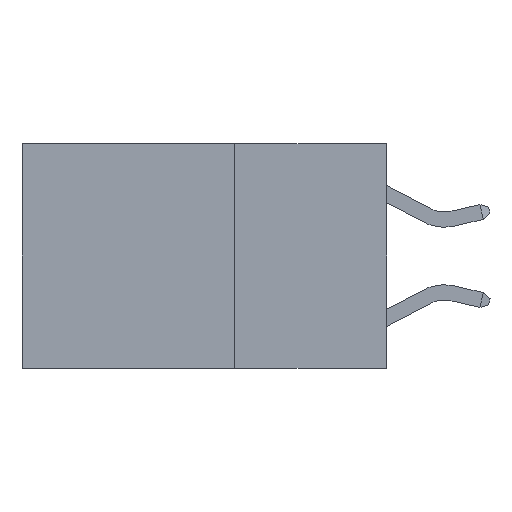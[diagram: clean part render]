
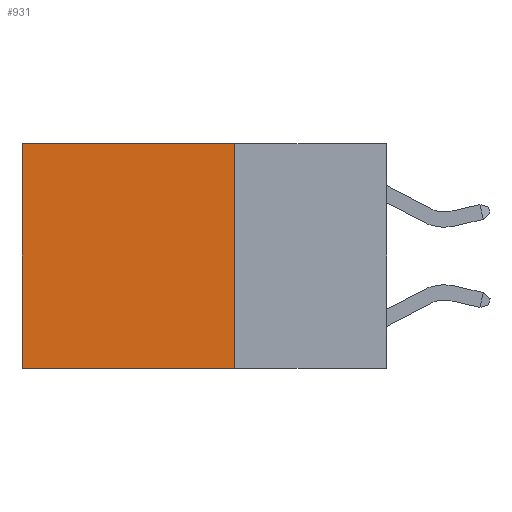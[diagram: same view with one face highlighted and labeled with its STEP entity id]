
A CAD part, left-side view. The second image highlights one B-rep face of the part: STEP entity #931.
In plain terms, the highlighted planar face has unit normal (-1, 0, 0).
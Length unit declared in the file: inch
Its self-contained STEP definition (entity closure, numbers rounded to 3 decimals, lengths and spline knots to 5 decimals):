
#561 = CARTESIAN_POINT ( 'NONE',  ( 0.2625, 0.25, 0. ) ) ;
#931 = ADVANCED_FACE ( 'NONE', ( #9192 ), #5574, .F. ) ;
#1033 = ORIENTED_EDGE ( 'NONE', *, *, #20461, .F. ) ;
#3840 = EDGE_CURVE ( 'NONE', #14281, #7035, #6710, .T. ) ;
#4538 = DIRECTION ( 'NONE',  ( 0., 0., -1. ) ) ;
#4697 = DIRECTION ( 'NONE',  ( 0., 0., -1. ) ) ;
#5280 = LINE ( 'NONE', #10106, #14316 ) ;
#5574 = PLANE ( 'NONE',  #21996 ) ;
#6447 = CARTESIAN_POINT ( 'NONE',  ( 0.2625, 0.25, 0. ) ) ;
#6710 = LINE ( 'NONE', #6447, #12651 ) ;
#7035 = VERTEX_POINT ( 'NONE', #10033 ) ;
#7344 = ORIENTED_EDGE ( 'NONE', *, *, #3840, .T. ) ;
#8641 = VECTOR ( 'NONE', #4538, 39.37008 ) ;
#9192 = FACE_OUTER_BOUND ( 'NONE', #16391, .T. ) ;
#10033 = CARTESIAN_POINT ( 'NONE',  ( 0.2625, 0.6, 0. ) ) ;
#10106 = CARTESIAN_POINT ( 'NONE',  ( 0.2625, 0.6, 0. ) ) ;
#10982 = DIRECTION ( 'NONE',  ( 1., 0., 0. ) ) ;
#12203 = CARTESIAN_POINT ( 'NONE',  ( 0.2625, 0.25, -0.37 ) ) ;
#12304 = VECTOR ( 'NONE', #15843, 39.37008 ) ;
#12651 = VECTOR ( 'NONE', #19013, 39.37008 ) ;
#13457 = LINE ( 'NONE', #561, #8641 ) ;
#14037 = CARTESIAN_POINT ( 'NONE',  ( 0.2625, 0.25, -0.37 ) ) ;
#14281 = VERTEX_POINT ( 'NONE', #15519 ) ;
#14316 = VECTOR ( 'NONE', #4697, 39.37008 ) ;
#15519 = CARTESIAN_POINT ( 'NONE',  ( 0.2625, 0.25, 0. ) ) ;
#15843 = DIRECTION ( 'NONE',  ( 0., 1., 0. ) ) ;
#16391 = EDGE_LOOP ( 'NONE', ( #23557, #19391, #1033, #7344 ) ) ;
#18128 = CARTESIAN_POINT ( 'NONE',  ( 0.2625, 0.25, 0. ) ) ;
#18464 = VERTEX_POINT ( 'NONE', #21581 ) ;
#19013 = DIRECTION ( 'NONE',  ( 0., 1., 0. ) ) ;
#19391 = ORIENTED_EDGE ( 'NONE', *, *, #21875, .F. ) ;
#20461 = EDGE_CURVE ( 'NONE', #14281, #22684, #13457, .T. ) ;
#20970 = EDGE_CURVE ( 'NONE', #7035, #18464, #5280, .T. ) ;
#21581 = CARTESIAN_POINT ( 'NONE',  ( 0.2625, 0.6, -0.37 ) ) ;
#21777 = LINE ( 'NONE', #14037, #12304 ) ;
#21875 = EDGE_CURVE ( 'NONE', #22684, #18464, #21777, .T. ) ;
#21996 = AXIS2_PLACEMENT_3D ( 'NONE', #18128, #10982, #23475 ) ;
#22684 = VERTEX_POINT ( 'NONE', #12203 ) ;
#23475 = DIRECTION ( 'NONE',  ( 0., 0., -1. ) ) ;
#23557 = ORIENTED_EDGE ( 'NONE', *, *, #20970, .T. ) ;
